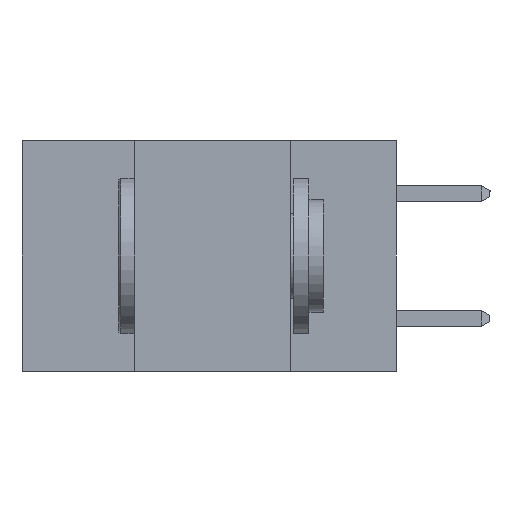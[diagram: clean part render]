
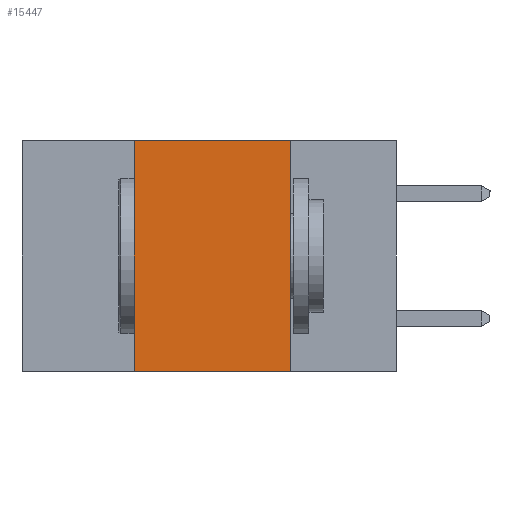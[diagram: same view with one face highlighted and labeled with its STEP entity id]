
A CAD part, left-side view. The second image highlights one B-rep face of the part: STEP entity #15447.
In plain terms, the highlighted planar face has unit normal (-1, 0, 0).
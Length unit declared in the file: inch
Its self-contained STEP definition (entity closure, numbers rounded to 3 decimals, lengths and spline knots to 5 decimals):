
#94 = CARTESIAN_POINT ( 'NONE',  ( 0., 0.17, 0. ) ) ;
#823 = DIRECTION ( 'NONE',  ( 0., 0., -1. ) ) ;
#831 = VERTEX_POINT ( 'NONE', #94 ) ;
#901 = DIRECTION ( 'NONE',  ( 0., -1., 0. ) ) ;
#977 = EDGE_LOOP ( 'NONE', ( #11872, #6911, #20442, #12161 ) ) ;
#2826 = DIRECTION ( 'NONE',  ( 1., 0., 0. ) ) ;
#3129 = VECTOR ( 'NONE', #17610, 39.37008 ) ;
#3361 = LINE ( 'NONE', #14903, #22500 ) ;
#6361 = EDGE_CURVE ( 'NONE', #24058, #9353, #10443, .T. ) ;
#6564 = CARTESIAN_POINT ( 'NONE',  ( 0., 0.42, -0.37 ) ) ;
#6911 = ORIENTED_EDGE ( 'NONE', *, *, #9243, .F. ) ;
#8666 = CARTESIAN_POINT ( 'NONE',  ( 0., 0.17, -0.37 ) ) ;
#8964 = LINE ( 'NONE', #22156, #14108 ) ;
#9243 = EDGE_CURVE ( 'NONE', #9771, #831, #9581, .T. ) ;
#9353 = VERTEX_POINT ( 'NONE', #8666 ) ;
#9581 = LINE ( 'NONE', #17237, #3129 ) ;
#9771 = VERTEX_POINT ( 'NONE', #23833 ) ;
#10169 = AXIS2_PLACEMENT_3D ( 'NONE', #20247, #2826, #823 ) ;
#10443 = LINE ( 'NONE', #19971, #13104 ) ;
#11872 = ORIENTED_EDGE ( 'NONE', *, *, #13417, .F. ) ;
#12161 = ORIENTED_EDGE ( 'NONE', *, *, #6361, .T. ) ;
#12591 = FACE_OUTER_BOUND ( 'NONE', #977, .T. ) ;
#13022 = DIRECTION ( 'NONE',  ( 0., 0., -1. ) ) ;
#13104 = VECTOR ( 'NONE', #901, 39.37008 ) ;
#13417 = EDGE_CURVE ( 'NONE', #831, #9353, #3361, .T. ) ;
#13778 = EDGE_CURVE ( 'NONE', #24058, #9771, #8964, .T. ) ;
#14108 = VECTOR ( 'NONE', #20270, 39.37008 ) ;
#14471 = PLANE ( 'NONE',  #10169 ) ;
#14903 = CARTESIAN_POINT ( 'NONE',  ( 0., 0.17, -0.37 ) ) ;
#15447 = ADVANCED_FACE ( 'NONE', ( #12591 ), #14471, .F. ) ;
#17237 = CARTESIAN_POINT ( 'NONE',  ( 0., 0.6, 0. ) ) ;
#17610 = DIRECTION ( 'NONE',  ( 0., -1., 0. ) ) ;
#19971 = CARTESIAN_POINT ( 'NONE',  ( 0., 0.6, -0.37 ) ) ;
#20247 = CARTESIAN_POINT ( 'NONE',  ( 0., 0.6, 0. ) ) ;
#20270 = DIRECTION ( 'NONE',  ( 0., 0., 1. ) ) ;
#20442 = ORIENTED_EDGE ( 'NONE', *, *, #13778, .F. ) ;
#22156 = CARTESIAN_POINT ( 'NONE',  ( 0., 0.42, -0.37 ) ) ;
#22500 = VECTOR ( 'NONE', #13022, 39.37008 ) ;
#23833 = CARTESIAN_POINT ( 'NONE',  ( 0., 0.42, 0. ) ) ;
#24058 = VERTEX_POINT ( 'NONE', #6564 ) ;
